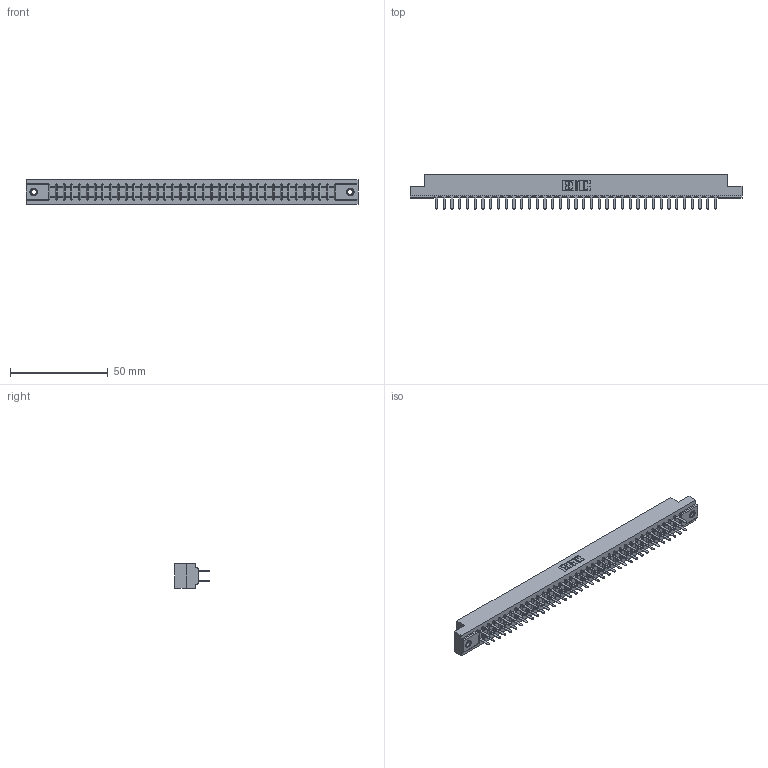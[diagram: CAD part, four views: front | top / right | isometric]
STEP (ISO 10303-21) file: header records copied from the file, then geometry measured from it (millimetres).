
FILE_DESCRIPTION (( 'STEP AP203' ), '1' );
FILE_NAME ('357-074-520-207.STEP', '2019-09-19T12:08:49', ( '' ), ( '' ), 'SwSTEP 2.0', 'SolidWorks 2016', '' );
FILE_SCHEMA (( 'CONFIG_CONTROL_DESIGN' ));
Length unit declared in the file: inch
Products named in the file (4): 307-290-001_520; 357-074-520-207; 345-250-001_345-250-005-103; 307 Part_.156 Dia Mounting Holes
Assembly tree (77 placements, depth 2):
  357-074-520-207
    307 Part_.156 Dia Mounting Holes
    307-290-001_520  x74
    345-250-001_345-250-005-103  x2
Bounding box: 169.62 x 17.42 x 12.7 mm (x, y, z)
Volume: 18042.5 mm3; surface area: 22127.3 mm2
Topology: 77 solids, 77 shells, 3620 faces, 10079 edges, 6510 vertices
Faces by surface type: plane 2396, cylinder 1132, sphere 76, cone 12, torus 4
Entity records: 34673 total; most frequent: CARTESIAN_POINT 5656, ORIENTED_EDGE 5598, DIRECTION 5551, EDGE_CURVE 2799, LINE 2145, VECTOR 2145, VERTEX_POINT 1808, AXIS2_PLACEMENT_3D 1703
